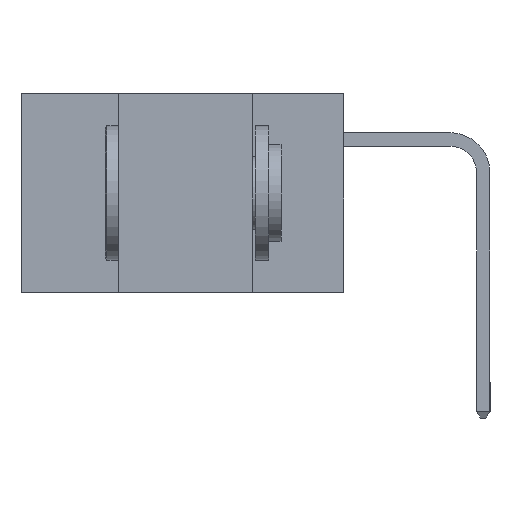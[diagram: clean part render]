
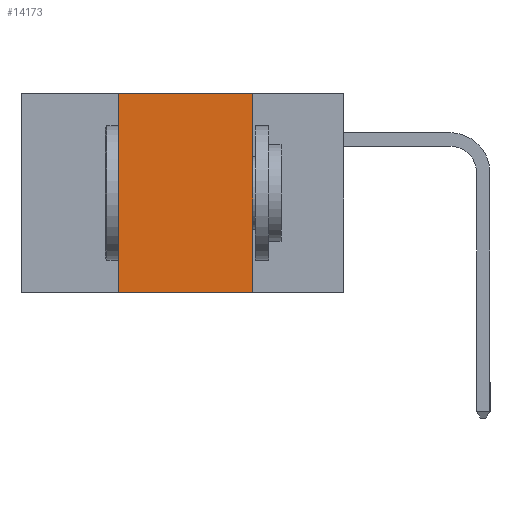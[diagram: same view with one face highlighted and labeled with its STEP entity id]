
A CAD part, left-side view. The second image highlights one B-rep face of the part: STEP entity #14173.
In plain terms, the highlighted planar face has unit normal (-1, 0, 0).
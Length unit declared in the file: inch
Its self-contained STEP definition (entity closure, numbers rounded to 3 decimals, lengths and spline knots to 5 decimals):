
#866 = CARTESIAN_POINT ( 'NONE',  ( 0., 0.42, 0. ) ) ;
#897 = FACE_OUTER_BOUND ( 'NONE', #9379, .T. ) ;
#1930 = DIRECTION ( 'NONE',  ( 0., -1., 0. ) ) ;
#2779 = DIRECTION ( 'NONE',  ( 0., 0., 1. ) ) ;
#3570 = EDGE_CURVE ( 'NONE', #20162, #19845, #10589, .T. ) ;
#3647 = VERTEX_POINT ( 'NONE', #866 ) ;
#3908 = ORIENTED_EDGE ( 'NONE', *, *, #3570, .T. ) ;
#4241 = VECTOR ( 'NONE', #18182, 39.37008 ) ;
#4832 = CARTESIAN_POINT ( 'NONE',  ( 0., 0.6, 0. ) ) ;
#6204 = VECTOR ( 'NONE', #1930, 39.37008 ) ;
#6819 = AXIS2_PLACEMENT_3D ( 'NONE', #4832, #17966, #8103 ) ;
#8103 = DIRECTION ( 'NONE',  ( 0., 0., -1. ) ) ;
#9379 = EDGE_LOOP ( 'NONE', ( #14227, #19500, #12125, #3908 ) ) ;
#9718 = PLANE ( 'NONE',  #6819 ) ;
#10233 = CARTESIAN_POINT ( 'NONE',  ( 0., 0.17, -0.37 ) ) ;
#10307 = CARTESIAN_POINT ( 'NONE',  ( 0., 0.17, 0. ) ) ;
#10335 = EDGE_CURVE ( 'NONE', #3647, #15433, #16159, .T. ) ;
#10589 = LINE ( 'NONE', #19188, #6204 ) ;
#10913 = CARTESIAN_POINT ( 'NONE',  ( 0., 0.42, 0. ) ) ;
#11177 = LINE ( 'NONE', #10913, #14580 ) ;
#12125 = ORIENTED_EDGE ( 'NONE', *, *, #16286, .F. ) ;
#12233 = EDGE_CURVE ( 'NONE', #15433, #19845, #12474, .T. ) ;
#12474 = LINE ( 'NONE', #14959, #4241 ) ;
#14173 = ADVANCED_FACE ( 'NONE', ( #897 ), #9718, .F. ) ;
#14227 = ORIENTED_EDGE ( 'NONE', *, *, #12233, .F. ) ;
#14357 = CARTESIAN_POINT ( 'NONE',  ( 0., 0.42, -0.37 ) ) ;
#14580 = VECTOR ( 'NONE', #2779, 39.37008 ) ;
#14959 = CARTESIAN_POINT ( 'NONE',  ( 0., 0.17, 0. ) ) ;
#15433 = VERTEX_POINT ( 'NONE', #10307 ) ;
#16159 = LINE ( 'NONE', #17315, #19892 ) ;
#16286 = EDGE_CURVE ( 'NONE', #20162, #3647, #11177, .T. ) ;
#17315 = CARTESIAN_POINT ( 'NONE',  ( 0., 0.6, 0. ) ) ;
#17966 = DIRECTION ( 'NONE',  ( 1., 0., 0. ) ) ;
#18182 = DIRECTION ( 'NONE',  ( 0., 0., -1. ) ) ;
#18908 = DIRECTION ( 'NONE',  ( 0., -1., 0. ) ) ;
#19188 = CARTESIAN_POINT ( 'NONE',  ( 0., 0.6, -0.37 ) ) ;
#19500 = ORIENTED_EDGE ( 'NONE', *, *, #10335, .F. ) ;
#19845 = VERTEX_POINT ( 'NONE', #10233 ) ;
#19892 = VECTOR ( 'NONE', #18908, 39.37008 ) ;
#20162 = VERTEX_POINT ( 'NONE', #14357 ) ;
